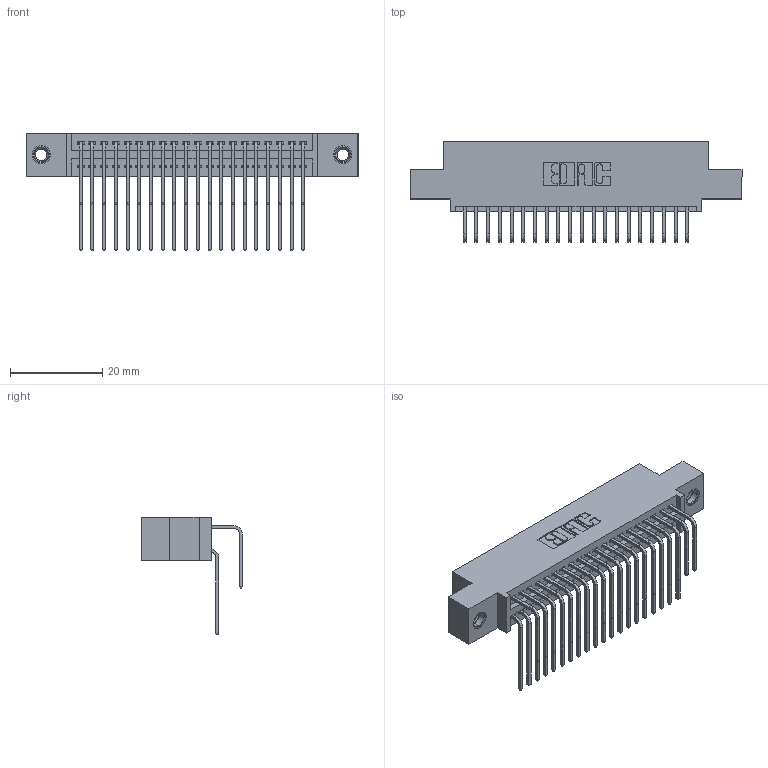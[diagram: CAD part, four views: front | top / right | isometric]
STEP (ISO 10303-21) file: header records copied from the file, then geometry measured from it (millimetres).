
FILE_DESCRIPTION (( 'STEP AP203' ), '1' );
FILE_NAME ('395-040-558-507.STEP', '2018-11-14T23:02:20', ( '' ), ( '' ), 'SwSTEP 2.0', 'SolidWorks 2016', '' );
FILE_SCHEMA (( 'CONFIG_CONTROL_DESIGN' ));
Length unit declared in the file: inch
Products named in the file (5): 345-292-001_558 Tail - 2; 345 Part_0.110 Offset - 0.156 Dia-TI; 345-292-001_558 559 Tail - 1; 395-040-558-507; 345-250-001_345-250-005-103
Assembly tree (43 placements, depth 2):
  395-040-558-507
    345 Part_0.110 Offset - 0.156 Dia-TI
    345-292-001_558 559 Tail - 1  x20
    345-292-001_558 Tail - 2  x20
    345-250-001_345-250-005-103  x2
Bounding box: 72.01 x 21.83 x 25.53 mm (x, y, z)
Volume: 6934.7 mm3; surface area: 11030.3 mm2
Topology: 43 solids, 43 shells, 2270 faces, 6689 edges, 4398 vertices
Faces by surface type: plane 1516, cylinder 738, cone 12, torus 4
Entity records: 21624 total; most frequent: CARTESIAN_POINT 3674, ORIENTED_EDGE 3550, DIRECTION 3265, EDGE_CURVE 1775, LINE 1503, VECTOR 1503, VERTEX_POINT 1176, AXIS2_PLACEMENT_3D 881
